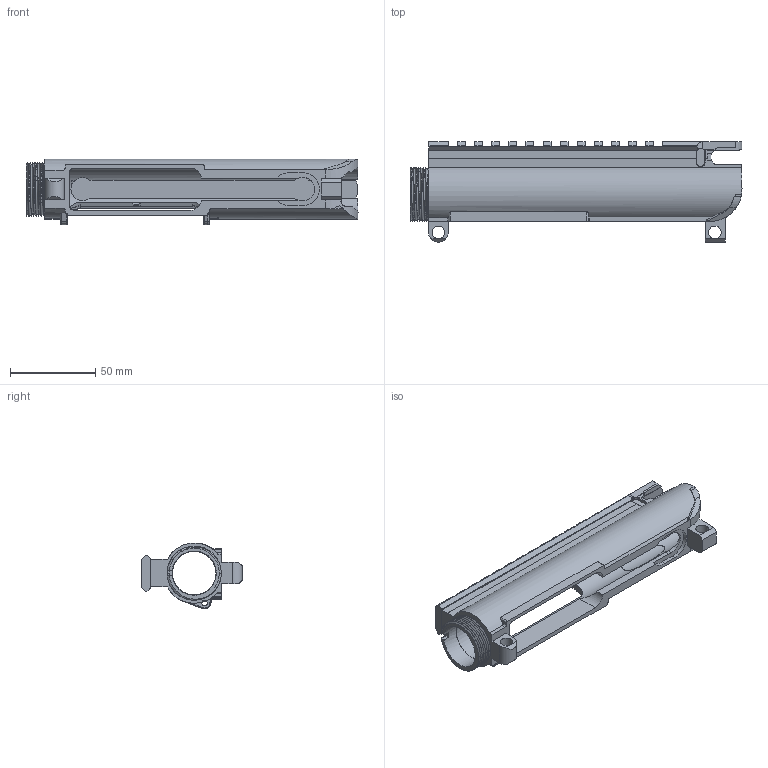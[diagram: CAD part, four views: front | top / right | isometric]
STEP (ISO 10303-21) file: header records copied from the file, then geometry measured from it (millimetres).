
FILE_DESCRIPTION(/* description */ (''),/* implementation_level */ '2;1');
FILE_NAME(/* name */ 'Upper Reciever - Daichi.step',/* time_stamp */ '2020-11-25T01:28:41-05:00',/* author */ (''),/* organization */ (''),/* preprocessor_version */ 'ST-DEVELOPER v18.1',/* originating_system */ 'Autodesk Translation Framework v9.3.0.1241',/* authorisation */ '');
FILE_SCHEMA (('AUTOMOTIVE_DESIGN { 1 0 10303 214 3 1 1 }'));
Length unit declared in the file: millimetre
Products named in the file (1): Upper Reciever - Daichi
Bounding box: 194.4 x 59 x 38.58 mm (x, y, z)
Volume: 79395.5 mm3; surface area: 49503.6 mm2
Topology: 1 solids, 2 shells, 452 faces, 1302 edges, 851 vertices
Faces by surface type: plane 254, cylinder 123, cone 48, bspline 15, torus 12
Full cylindrical faces by diameter (mm): 3.175 x2, 7.35 x1, 7.358 x1, 25.546 x1, 25.927 x1, 29.782 x1, 31.7 x4
Entity records: 18291 total; most frequent: CARTESIAN_POINT 6600, ORIENTED_EDGE 2602, DIRECTION 2251, EDGE_CURVE 1301, VERTEX_POINT 851, LINE 813, VECTOR 813, AXIS2_PLACEMENT_3D 719
